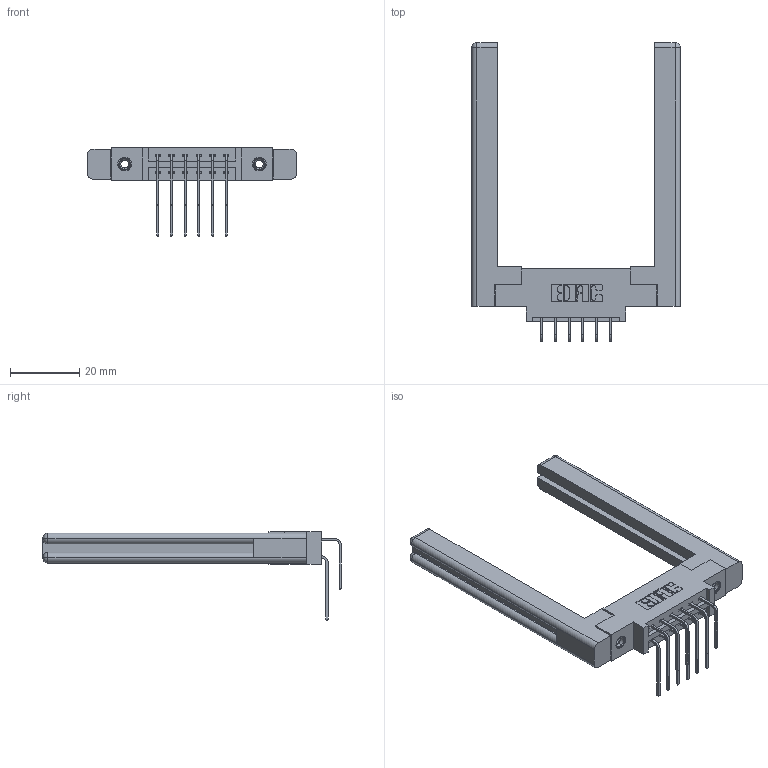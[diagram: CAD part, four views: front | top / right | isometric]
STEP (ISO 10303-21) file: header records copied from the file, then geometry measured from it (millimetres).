
FILE_DESCRIPTION (( 'STEP AP203' ), '1' );
FILE_NAME ('387-012-559-858.STEP', '2019-10-15T20:37:46', ( '' ), ( '' ), 'SwSTEP 2.0', 'SolidWorks 2016', '' );
FILE_SCHEMA (( 'CONFIG_CONTROL_DESIGN' ));
Length unit declared in the file: inch
Products named in the file (6): 345-292-001_559 Tail - 2; 345-250-001_345-250-001-102; 387-012-559-858; 345-292-001_558 559 Tail - 1; 337 Part_0.170 Offset - 0.156 Dia-TI; 307-220-058
Assembly tree (17 placements, depth 2):
  387-012-559-858
    337 Part_0.170 Offset - 0.156 Dia-TI
    345-292-001_558 559 Tail - 1  x6
    345-292-001_559 Tail - 2  x6
    345-250-001_345-250-001-102  x2
    307-220-058  x2
Bounding box: 60.4 x 86.3 x 25.53 mm (x, y, z)
Volume: 12980.4 mm3; surface area: 11752.4 mm2
Topology: 17 solids, 17 shells, 932 faces, 2681 edges, 1758 vertices
Faces by surface type: plane 638, cylinder 270, cone 12, torus 12
Entity records: 13858 total; most frequent: CARTESIAN_POINT 2420, ORIENTED_EDGE 2244, DIRECTION 2122, EDGE_CURVE 1122, VECTOR 906, LINE 906, VERTEX_POINT 738, AXIS2_PLACEMENT_3D 608
